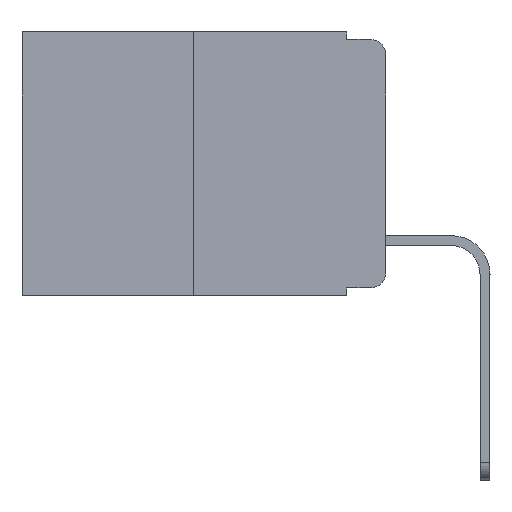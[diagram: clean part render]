
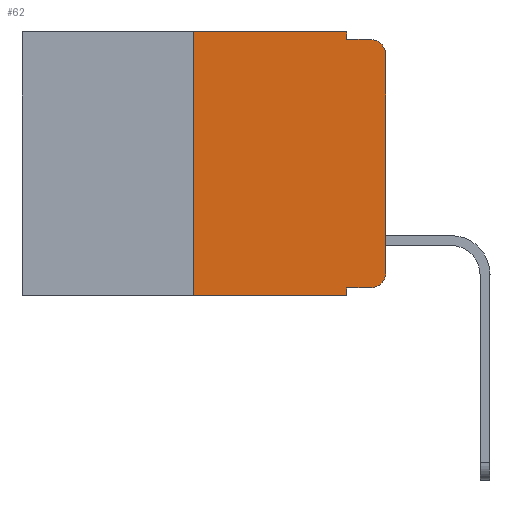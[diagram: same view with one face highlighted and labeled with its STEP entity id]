
A CAD part, left-side view. The second image highlights one B-rep face of the part: STEP entity #62.
In plain terms, the highlighted planar face has unit normal (-1, 0, 0).
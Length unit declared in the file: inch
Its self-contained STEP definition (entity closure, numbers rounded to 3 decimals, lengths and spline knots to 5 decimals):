
#62 = ADVANCED_FACE ( 'NONE', ( #964 ), #15155, .F. ) ;
#127 = VERTEX_POINT ( 'NONE', #16967 ) ;
#691 = VECTOR ( 'NONE', #11432, 39.37008 ) ;
#964 = FACE_OUTER_BOUND ( 'NONE', #4063, .T. ) ;
#1172 = EDGE_CURVE ( 'NONE', #4698, #14549, #18889, .T. ) ;
#1517 = DIRECTION ( 'NONE',  ( -1., 0., 0. ) ) ;
#1536 = AXIS2_PLACEMENT_3D ( 'NONE', #15217, #11945, #15078 ) ;
#1599 = CARTESIAN_POINT ( 'NONE',  ( 0., 0.473, -0.343 ) ) ;
#1642 = CIRCLE ( 'NONE', #3170, 0.02 ) ;
#1833 = CARTESIAN_POINT ( 'NONE',  ( 0., 0.051, -0.333 ) ) ;
#2114 = ORIENTED_EDGE ( 'NONE', *, *, #6968, .F. ) ;
#2403 = CARTESIAN_POINT ( 'NONE',  ( 0., 0.051, -0.343 ) ) ;
#2652 = EDGE_CURVE ( 'NONE', #9203, #12262, #9829, .T. ) ;
#2693 = CARTESIAN_POINT ( 'NONE',  ( 0., 0.25, 0. ) ) ;
#3170 = AXIS2_PLACEMENT_3D ( 'NONE', #17127, #6018, #17051 ) ;
#3470 = VERTEX_POINT ( 'NONE', #16101 ) ;
#4063 = EDGE_LOOP ( 'NONE', ( #14896, #12157, #7481, #5047, #15929, #2114, #9145, #19576, #19930, #5393 ) ) ;
#4120 = DIRECTION ( 'NONE',  ( 0., 0., -1. ) ) ;
#4698 = VERTEX_POINT ( 'NONE', #13716 ) ;
#4864 = CARTESIAN_POINT ( 'NONE',  ( 0., 0.051, 0. ) ) ;
#4896 = CARTESIAN_POINT ( 'NONE',  ( 0., 0.02, -0.333 ) ) ;
#5047 = ORIENTED_EDGE ( 'NONE', *, *, #9911, .F. ) ;
#5393 = ORIENTED_EDGE ( 'NONE', *, *, #2652, .T. ) ;
#5398 = DIRECTION ( 'NONE',  ( 0., -1., 0. ) ) ;
#6018 = DIRECTION ( 'NONE',  ( -1., 0., 0. ) ) ;
#6334 = EDGE_CURVE ( 'NONE', #127, #8115, #15390, .T. ) ;
#6740 = DIRECTION ( 'NONE',  ( 0., 0., 1. ) ) ;
#6854 = CARTESIAN_POINT ( 'NONE',  ( 0., 0.051, -0.01 ) ) ;
#6968 = EDGE_CURVE ( 'NONE', #127, #3470, #13151, .T. ) ;
#7323 = CARTESIAN_POINT ( 'NONE',  ( 0., 0., -0.313 ) ) ;
#7481 = ORIENTED_EDGE ( 'NONE', *, *, #1172, .F. ) ;
#8074 = LINE ( 'NONE', #19567, #16706 ) ;
#8115 = VERTEX_POINT ( 'NONE', #2403 ) ;
#8945 = VECTOR ( 'NONE', #16734, 39.37008 ) ;
#9110 = EDGE_CURVE ( 'NONE', #17332, #9203, #11499, .T. ) ;
#9145 = ORIENTED_EDGE ( 'NONE', *, *, #6334, .T. ) ;
#9203 = VERTEX_POINT ( 'NONE', #4896 ) ;
#9722 = VECTOR ( 'NONE', #11897, 39.37008 ) ;
#9829 = CIRCLE ( 'NONE', #15501, 0.02 ) ;
#9911 = EDGE_CURVE ( 'NONE', #10681, #4698, #15617, .T. ) ;
#10529 = VERTEX_POINT ( 'NONE', #12431 ) ;
#10619 = VECTOR ( 'NONE', #6740, 39.37008 ) ;
#10681 = VERTEX_POINT ( 'NONE', #4864 ) ;
#10931 = LINE ( 'NONE', #13545, #17335 ) ;
#11079 = EDGE_CURVE ( 'NONE', #3470, #10681, #10931, .T. ) ;
#11178 = CARTESIAN_POINT ( 'NONE',  ( 0., 0.02, -0.313 ) ) ;
#11432 = DIRECTION ( 'NONE',  ( 0., -1., 0. ) ) ;
#11499 = LINE ( 'NONE', #1833, #691 ) ;
#11897 = DIRECTION ( 'NONE',  ( 0., 0., -1. ) ) ;
#11945 = DIRECTION ( 'NONE',  ( 1., 0., 0. ) ) ;
#12157 = ORIENTED_EDGE ( 'NONE', *, *, #15669, .T. ) ;
#12262 = VERTEX_POINT ( 'NONE', #7323 ) ;
#12431 = CARTESIAN_POINT ( 'NONE',  ( 0., 0., -0.03 ) ) ;
#12510 = DIRECTION ( 'NONE',  ( 0., -1., 0. ) ) ;
#13151 = LINE ( 'NONE', #2693, #8945 ) ;
#13159 = CARTESIAN_POINT ( 'NONE',  ( 0., 0., 0. ) ) ;
#13545 = CARTESIAN_POINT ( 'NONE',  ( 0., 0.473, 0. ) ) ;
#13716 = CARTESIAN_POINT ( 'NONE',  ( 0., 0.051, -0.01 ) ) ;
#13973 = EDGE_CURVE ( 'NONE', #17332, #8115, #8074, .T. ) ;
#14407 = VECTOR ( 'NONE', #12510, 39.37008 ) ;
#14549 = VERTEX_POINT ( 'NONE', #19543 ) ;
#14896 = ORIENTED_EDGE ( 'NONE', *, *, #18269, .T. ) ;
#15029 = CARTESIAN_POINT ( 'NONE',  ( 0., 0.051, 0. ) ) ;
#15078 = DIRECTION ( 'NONE',  ( 0., 0., -1. ) ) ;
#15155 = PLANE ( 'NONE',  #1536 ) ;
#15217 = CARTESIAN_POINT ( 'NONE',  ( 0., 0.473, 0. ) ) ;
#15380 = VECTOR ( 'NONE', #5398, 39.37008 ) ;
#15390 = LINE ( 'NONE', #1599, #14407 ) ;
#15501 = AXIS2_PLACEMENT_3D ( 'NONE', #11178, #1517, #17303 ) ;
#15617 = LINE ( 'NONE', #15029, #9722 ) ;
#15669 = EDGE_CURVE ( 'NONE', #10529, #14549, #1642, .T. ) ;
#15929 = ORIENTED_EDGE ( 'NONE', *, *, #11079, .F. ) ;
#16101 = CARTESIAN_POINT ( 'NONE',  ( 0., 0.25, 0. ) ) ;
#16706 = VECTOR ( 'NONE', #4120, 39.37008 ) ;
#16734 = DIRECTION ( 'NONE',  ( 0., 0., 1. ) ) ;
#16851 = CARTESIAN_POINT ( 'NONE',  ( 0., 0.051, -0.333 ) ) ;
#16967 = CARTESIAN_POINT ( 'NONE',  ( 0., 0.25, -0.343 ) ) ;
#17051 = DIRECTION ( 'NONE',  ( 0., 0., -1. ) ) ;
#17127 = CARTESIAN_POINT ( 'NONE',  ( 0., 0.02, -0.03 ) ) ;
#17303 = DIRECTION ( 'NONE',  ( 0., 0., -1. ) ) ;
#17332 = VERTEX_POINT ( 'NONE', #16851 ) ;
#17335 = VECTOR ( 'NONE', #18207, 39.37008 ) ;
#18207 = DIRECTION ( 'NONE',  ( 0., -1., 0. ) ) ;
#18269 = EDGE_CURVE ( 'NONE', #12262, #10529, #19027, .T. ) ;
#18889 = LINE ( 'NONE', #6854, #15380 ) ;
#19027 = LINE ( 'NONE', #13159, #10619 ) ;
#19543 = CARTESIAN_POINT ( 'NONE',  ( 0., 0.02, -0.01 ) ) ;
#19567 = CARTESIAN_POINT ( 'NONE',  ( 0., 0.051, 0. ) ) ;
#19576 = ORIENTED_EDGE ( 'NONE', *, *, #13973, .F. ) ;
#19930 = ORIENTED_EDGE ( 'NONE', *, *, #9110, .T. ) ;
